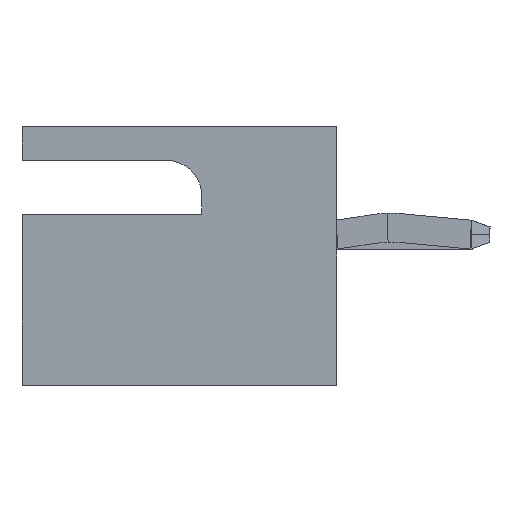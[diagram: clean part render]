
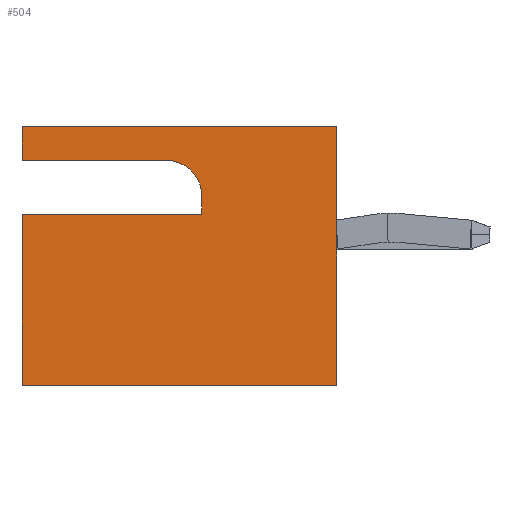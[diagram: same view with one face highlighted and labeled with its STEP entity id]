
A CAD part, left-side view. The second image highlights one B-rep face of the part: STEP entity #504.
In plain terms, the highlighted planar face has unit normal (-1, 0, 0).
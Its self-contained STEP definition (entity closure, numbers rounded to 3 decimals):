
#163 = EDGE_CURVE ( 'NONE', #3057, #6865, #8431, .T. ) ;
#241 = ORIENTED_EDGE ( 'NONE', *, *, #7182, .F. ) ;
#384 = CARTESIAN_POINT ( 'NONE',  ( -21.25, 7., 0.925 ) ) ;
#504 = ADVANCED_FACE ( 'NONE', ( #1376 ), #8194, .F. ) ;
#541 = CARTESIAN_POINT ( 'NONE',  ( -21.25, 7., -2.875 ) ) ;
#566 = EDGE_CURVE ( 'NONE', #1754, #7616, #1640, .T. ) ;
#604 = ORIENTED_EDGE ( 'NONE', *, *, #4757, .T. ) ;
#677 = VECTOR ( 'NONE', #1103, 1000. ) ;
#993 = ORIENTED_EDGE ( 'NONE', *, *, #566, .T. ) ;
#1020 = DIRECTION ( 'NONE',  ( 0., -1., 0. ) ) ;
#1103 = DIRECTION ( 'NONE',  ( 0., -1., 0. ) ) ;
#1376 = FACE_OUTER_BOUND ( 'NONE', #7411, .T. ) ;
#1544 = EDGE_CURVE ( 'NONE', #6836, #2798, #5124, .T. ) ;
#1622 = CARTESIAN_POINT ( 'NONE',  ( -21.25, 7., -2.875 ) ) ;
#1628 = CARTESIAN_POINT ( 'NONE',  ( -21.25, 7., -2.875 ) ) ;
#1640 = CIRCLE ( 'NONE', #7387, 0.8 ) ;
#1676 = CARTESIAN_POINT ( 'NONE',  ( -21.25, 0., -2.875 ) ) ;
#1739 = VECTOR ( 'NONE', #1020, 1000. ) ;
#1741 = DIRECTION ( 'NONE',  ( 0., 1., 0. ) ) ;
#1754 = VERTEX_POINT ( 'NONE', #8877 ) ;
#1885 = DIRECTION ( 'NONE',  ( 1., 0., 0. ) ) ;
#1926 = DIRECTION ( 'NONE',  ( 0., 0., -1. ) ) ;
#1962 = CARTESIAN_POINT ( 'NONE',  ( -21.25, 7., 2.125 ) ) ;
#2132 = VERTEX_POINT ( 'NONE', #4857 ) ;
#2300 = VECTOR ( 'NONE', #5830, 1000. ) ;
#2348 = LINE ( 'NONE', #3110, #1739 ) ;
#2403 = DIRECTION ( 'NONE',  ( 0., -1., 0. ) ) ;
#2422 = CARTESIAN_POINT ( 'NONE',  ( -21.25, 3., 1.325 ) ) ;
#2685 = LINE ( 'NONE', #541, #7450 ) ;
#2789 = EDGE_CURVE ( 'NONE', #3057, #6836, #4473, .T. ) ;
#2798 = VERTEX_POINT ( 'NONE', #6400 ) ;
#3057 = VERTEX_POINT ( 'NONE', #6425 ) ;
#3110 = CARTESIAN_POINT ( 'NONE',  ( -21.25, 7., 2.875 ) ) ;
#3276 = EDGE_CURVE ( 'NONE', #7616, #3892, #4455, .T. ) ;
#3565 = VERTEX_POINT ( 'NONE', #4526 ) ;
#3605 = ORIENTED_EDGE ( 'NONE', *, *, #3276, .T. ) ;
#3816 = EDGE_CURVE ( 'NONE', #2132, #3565, #2685, .T. ) ;
#3892 = VERTEX_POINT ( 'NONE', #5507 ) ;
#3909 = LINE ( 'NONE', #8087, #7934 ) ;
#4036 = VECTOR ( 'NONE', #7913, 1000. ) ;
#4128 = ORIENTED_EDGE ( 'NONE', *, *, #163, .F. ) ;
#4142 = CARTESIAN_POINT ( 'NONE',  ( -21.25, 7., -2.875 ) ) ;
#4197 = ORIENTED_EDGE ( 'NONE', *, *, #2789, .T. ) ;
#4407 = CARTESIAN_POINT ( 'NONE',  ( -21.25, 3., 1.325 ) ) ;
#4455 = LINE ( 'NONE', #2422, #4036 ) ;
#4472 = ORIENTED_EDGE ( 'NONE', *, *, #1544, .T. ) ;
#4473 = LINE ( 'NONE', #1622, #5206 ) ;
#4526 = CARTESIAN_POINT ( 'NONE',  ( -21.25, 7., 2.875 ) ) ;
#4757 = EDGE_CURVE ( 'NONE', #2132, #1754, #7283, .T. ) ;
#4857 = CARTESIAN_POINT ( 'NONE',  ( -21.25, 7., 2.125 ) ) ;
#5124 = LINE ( 'NONE', #1676, #2300 ) ;
#5206 = VECTOR ( 'NONE', #2403, 1000. ) ;
#5507 = CARTESIAN_POINT ( 'NONE',  ( -21.25, 3., 0.925 ) ) ;
#5830 = DIRECTION ( 'NONE',  ( 0., 0., 1. ) ) ;
#5893 = ORIENTED_EDGE ( 'NONE', *, *, #3816, .F. ) ;
#6400 = CARTESIAN_POINT ( 'NONE',  ( -21.25, 0., 2.875 ) ) ;
#6425 = CARTESIAN_POINT ( 'NONE',  ( -21.25, 7., -2.875 ) ) ;
#6621 = ORIENTED_EDGE ( 'NONE', *, *, #7339, .T. ) ;
#6836 = VERTEX_POINT ( 'NONE', #8053 ) ;
#6865 = VERTEX_POINT ( 'NONE', #384 ) ;
#7169 = DIRECTION ( 'NONE',  ( 0., 0., 1. ) ) ;
#7182 = EDGE_CURVE ( 'NONE', #3565, #2798, #2348, .T. ) ;
#7283 = LINE ( 'NONE', #1962, #677 ) ;
#7339 = EDGE_CURVE ( 'NONE', #3892, #6865, #3909, .T. ) ;
#7387 = AXIS2_PLACEMENT_3D ( 'NONE', #8102, #8151, #1926 ) ;
#7411 = EDGE_LOOP ( 'NONE', ( #5893, #604, #993, #3605, #6621, #4128, #4197, #4472, #241 ) ) ;
#7450 = VECTOR ( 'NONE', #8208, 1000. ) ;
#7515 = DIRECTION ( 'NONE',  ( 0., 0., -1. ) ) ;
#7616 = VERTEX_POINT ( 'NONE', #4407 ) ;
#7681 = AXIS2_PLACEMENT_3D ( 'NONE', #4142, #1885, #7515 ) ;
#7913 = DIRECTION ( 'NONE',  ( 0., 0., -1. ) ) ;
#7934 = VECTOR ( 'NONE', #1741, 1000. ) ;
#8053 = CARTESIAN_POINT ( 'NONE',  ( -21.25, 0., -2.875 ) ) ;
#8087 = CARTESIAN_POINT ( 'NONE',  ( -21.25, 7., 0.925 ) ) ;
#8102 = CARTESIAN_POINT ( 'NONE',  ( -21.25, 3.8, 1.325 ) ) ;
#8151 = DIRECTION ( 'NONE',  ( 1., 0., 0. ) ) ;
#8194 = PLANE ( 'NONE',  #7681 ) ;
#8208 = DIRECTION ( 'NONE',  ( 0., 0., 1. ) ) ;
#8431 = LINE ( 'NONE', #1628, #8670 ) ;
#8670 = VECTOR ( 'NONE', #7169, 1000. ) ;
#8877 = CARTESIAN_POINT ( 'NONE',  ( -21.25, 3.8, 2.125 ) ) ;
